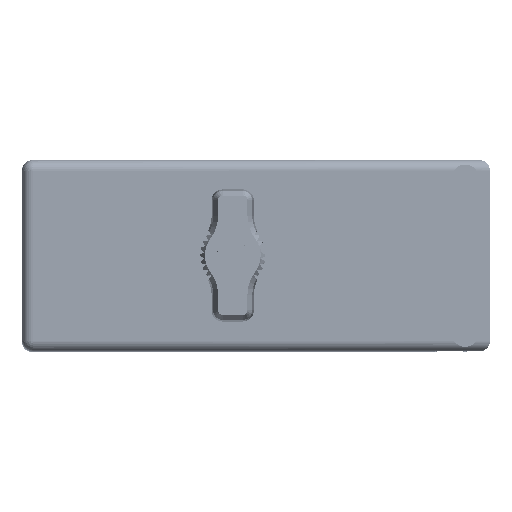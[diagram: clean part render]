
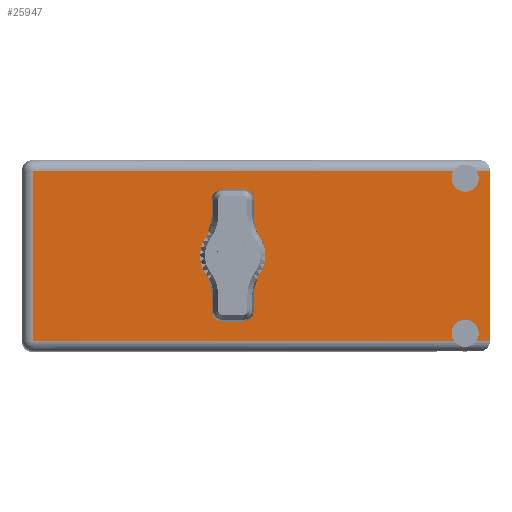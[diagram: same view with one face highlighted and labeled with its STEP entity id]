
A CAD part, top view. The second image highlights one B-rep face of the part: STEP entity #25947.
In plain terms, the highlighted face is planar.
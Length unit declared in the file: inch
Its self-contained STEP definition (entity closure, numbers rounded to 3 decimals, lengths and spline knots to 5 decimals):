
#608 = EDGE_CURVE ( 'NONE', #64827, #43503, #43738, .T. ) ;
#1348 = ORIENTED_EDGE ( 'NONE', *, *, #72574, .F. ) ;
#2503 = CARTESIAN_POINT ( 'NONE',  ( 2.858, 1.775, -1.117 ) ) ;
#2552 = EDGE_CURVE ( 'NONE', #55815, #45281, #53048, .T. ) ;
#5391 = EDGE_CURVE ( 'NONE', #49593, #26605, #30068, .T. ) ;
#7016 = CARTESIAN_POINT ( 'NONE',  ( 1.359, 1.775, -0.742 ) ) ;
#7832 = VERTEX_POINT ( 'NONE', #7016 ) ;
#7969 = DIRECTION ( 'NONE',  ( 0., 1., 0. ) ) ;
#9832 = DIRECTION ( 'NONE',  ( 0., 0., 1. ) ) ;
#10284 = CARTESIAN_POINT ( 'NONE',  ( 3.018, 1.775, -0.07 ) ) ;
#10767 = DIRECTION ( 'NONE',  ( 0., 1., 0. ) ) ;
#10955 = CARTESIAN_POINT ( 'NONE',  ( 2.78419, 1.775, -0.07 ) ) ;
#11032 = CARTESIAN_POINT ( 'NONE',  ( 0., 1.775, -1.164 ) ) ;
#12153 = VERTEX_POINT ( 'NONE', #41009 ) ;
#12749 = LINE ( 'NONE', #25932, #21412 ) ;
#14226 = VERTEX_POINT ( 'NONE', #76802 ) ;
#15541 = CARTESIAN_POINT ( 'NONE',  ( 0., 1.775, -1.234 ) ) ;
#15867 = EDGE_LOOP ( 'NONE', ( #76653, #56327, #40020, #50385, #50510, #75709, #87005, #17679, #46593, #50415 ) ) ;
#16666 = CARTESIAN_POINT ( 'NONE',  ( 2.858, 1.775, -1.117 ) ) ;
#17679 = ORIENTED_EDGE ( 'NONE', *, *, #23216, .F. ) ;
#18230 = DIRECTION ( 'NONE',  ( 0., 0., 1. ) ) ;
#19751 = CARTESIAN_POINT ( 'NONE',  ( 2.858, 1.775, -0.2045 ) ) ;
#20551 = LINE ( 'NONE', #66817, #37761 ) ;
#21412 = VECTOR ( 'NONE', #59395, 39.37008 ) ;
#21891 = AXIS2_PLACEMENT_3D ( 'NONE', #16666, #84684, #18230 ) ;
#21928 = DIRECTION ( 'NONE',  ( 0., 0., 1. ) ) ;
#22637 = AXIS2_PLACEMENT_3D ( 'NONE', #57628, #30516, #30221 ) ;
#22793 = VERTEX_POINT ( 'NONE', #72732 ) ;
#23216 = EDGE_CURVE ( 'NONE', #35299, #14226, #62063, .T. ) ;
#23480 = CARTESIAN_POINT ( 'NONE',  ( 0.07, 1.775, -0.07 ) ) ;
#23585 = CARTESIAN_POINT ( 'NONE',  ( 1.359, 1.775, -0.617 ) ) ;
#23761 = CARTESIAN_POINT ( 'NONE',  ( 3.018, 1.775, -0.07 ) ) ;
#23885 = DIRECTION ( 'NONE',  ( 0., 1., 0. ) ) ;
#24625 = DIRECTION ( 'NONE',  ( -1., 0., 0. ) ) ;
#24783 = EDGE_CURVE ( 'NONE', #35299, #22793, #45577, .T. ) ;
#25428 = CARTESIAN_POINT ( 'NONE',  ( 3.018, 1.775, -0.07 ) ) ;
#25932 = CARTESIAN_POINT ( 'NONE',  ( 0.07, 1.775, -1.234 ) ) ;
#25947 = ADVANCED_FACE ( 'NONE', ( #63700, #45318 ), #55640, .T. ) ;
#26605 = VERTEX_POINT ( 'NONE', #72598 ) ;
#26608 = CARTESIAN_POINT ( 'NONE',  ( 0., 1.775, -1.164 ) ) ;
#27994 = EDGE_CURVE ( 'NONE', #7832, #12153, #41611, .T. ) ;
#30068 = LINE ( 'NONE', #26608, #33294 ) ;
#30221 = DIRECTION ( 'NONE',  ( 0., 0., 1. ) ) ;
#30516 = DIRECTION ( 'NONE',  ( 0., 1., 0. ) ) ;
#31467 = AXIS2_PLACEMENT_3D ( 'NONE', #60810, #88711, #53539 ) ;
#32338 = DIRECTION ( 'NONE',  ( 1., 0., 0. ) ) ;
#32915 = CIRCLE ( 'NONE', #31467, 0.125 ) ;
#33294 = VECTOR ( 'NONE', #47387, 39.37008 ) ;
#33618 = CIRCLE ( 'NONE', #22637, 0.0875 ) ;
#35299 = VERTEX_POINT ( 'NONE', #47655 ) ;
#35574 = EDGE_LOOP ( 'NONE', ( #1348, #53172 ) ) ;
#36454 = CARTESIAN_POINT ( 'NONE',  ( 2.93181, 1.775, -0.07 ) ) ;
#37761 = VECTOR ( 'NONE', #59863, 39.37008 ) ;
#37840 = VERTEX_POINT ( 'NONE', #19751 ) ;
#40020 = ORIENTED_EDGE ( 'NONE', *, *, #79323, .F. ) ;
#41009 = CARTESIAN_POINT ( 'NONE',  ( 1.359, 1.775, -0.492 ) ) ;
#41571 = EDGE_CURVE ( 'NONE', #14226, #26605, #48069, .T. ) ;
#41611 = CIRCLE ( 'NONE', #65567, 0.125 ) ;
#42751 = EDGE_CURVE ( 'NONE', #37840, #43503, #49966, .T. ) ;
#43496 = DIRECTION ( 'NONE',  ( 0., 0., 1. ) ) ;
#43503 = VERTEX_POINT ( 'NONE', #10955 ) ;
#43738 = LINE ( 'NONE', #10284, #52410 ) ;
#45281 = VERTEX_POINT ( 'NONE', #23761 ) ;
#45318 = FACE_OUTER_BOUND ( 'NONE', #15867, .T. ) ;
#45577 = LINE ( 'NONE', #11032, #68267 ) ;
#46593 = ORIENTED_EDGE ( 'NONE', *, *, #24783, .T. ) ;
#47387 = DIRECTION ( 'NONE',  ( -1., 0., 0. ) ) ;
#47655 = CARTESIAN_POINT ( 'NONE',  ( 2.78419, 1.775, -1.164 ) ) ;
#48069 = CIRCLE ( 'NONE', #21891, 0.0875 ) ;
#49593 = VERTEX_POINT ( 'NONE', #88705 ) ;
#49966 = CIRCLE ( 'NONE', #69245, 0.0875 ) ;
#50385 = ORIENTED_EDGE ( 'NONE', *, *, #2552, .T. ) ;
#50415 = ORIENTED_EDGE ( 'NONE', *, *, #54622, .T. ) ;
#50510 = ORIENTED_EDGE ( 'NONE', *, *, #69260, .F. ) ;
#51152 = CARTESIAN_POINT ( 'NONE',  ( 2.858, 1.775, -0.117 ) ) ;
#52410 = VECTOR ( 'NONE', #32338, 39.37008 ) ;
#53048 = LINE ( 'NONE', #25428, #55197 ) ;
#53172 = ORIENTED_EDGE ( 'NONE', *, *, #27994, .F. ) ;
#53539 = DIRECTION ( 'NONE',  ( 0., 0., 1. ) ) ;
#54622 = EDGE_CURVE ( 'NONE', #22793, #64827, #12749, .T. ) ;
#55197 = VECTOR ( 'NONE', #81029, 39.37008 ) ;
#55640 = PLANE ( 'NONE',  #71692 ) ;
#55815 = VERTEX_POINT ( 'NONE', #36454 ) ;
#56327 = ORIENTED_EDGE ( 'NONE', *, *, #42751, .F. ) ;
#57082 = DIRECTION ( 'NONE',  ( 0., 1., 0. ) ) ;
#57628 = CARTESIAN_POINT ( 'NONE',  ( 2.858, 1.775, -0.117 ) ) ;
#59395 = DIRECTION ( 'NONE',  ( 0., 0., 1. ) ) ;
#59863 = DIRECTION ( 'NONE',  ( 0., 0., 1. ) ) ;
#60810 = CARTESIAN_POINT ( 'NONE',  ( 1.359, 1.775, -0.617 ) ) ;
#62063 = CIRCLE ( 'NONE', #79567, 0.0875 ) ;
#63700 = FACE_BOUND ( 'NONE', #35574, .T. ) ;
#64827 = VERTEX_POINT ( 'NONE', #23480 ) ;
#65567 = AXIS2_PLACEMENT_3D ( 'NONE', #23585, #23885, #85229 ) ;
#66817 = CARTESIAN_POINT ( 'NONE',  ( 3.018, 1.775, 0. ) ) ;
#68267 = VECTOR ( 'NONE', #24625, 39.37008 ) ;
#69245 = AXIS2_PLACEMENT_3D ( 'NONE', #51152, #10767, #9832 ) ;
#69260 = EDGE_CURVE ( 'NONE', #49593, #45281, #20551, .T. ) ;
#71692 = AXIS2_PLACEMENT_3D ( 'NONE', #15541, #7969, #21928 ) ;
#72574 = EDGE_CURVE ( 'NONE', #12153, #7832, #32915, .T. ) ;
#72598 = CARTESIAN_POINT ( 'NONE',  ( 2.93181, 1.775, -1.164 ) ) ;
#72732 = CARTESIAN_POINT ( 'NONE',  ( 0.07, 1.775, -1.164 ) ) ;
#75709 = ORIENTED_EDGE ( 'NONE', *, *, #5391, .T. ) ;
#76653 = ORIENTED_EDGE ( 'NONE', *, *, #608, .T. ) ;
#76802 = CARTESIAN_POINT ( 'NONE',  ( 2.858, 1.775, -1.0295 ) ) ;
#79323 = EDGE_CURVE ( 'NONE', #55815, #37840, #33618, .T. ) ;
#79567 = AXIS2_PLACEMENT_3D ( 'NONE', #2503, #57082, #43496 ) ;
#81029 = DIRECTION ( 'NONE',  ( 1., 0., 0. ) ) ;
#84684 = DIRECTION ( 'NONE',  ( 0., 1., 0. ) ) ;
#85229 = DIRECTION ( 'NONE',  ( 0., 0., 1. ) ) ;
#87005 = ORIENTED_EDGE ( 'NONE', *, *, #41571, .F. ) ;
#88705 = CARTESIAN_POINT ( 'NONE',  ( 3.018, 1.775, -1.164 ) ) ;
#88711 = DIRECTION ( 'NONE',  ( 0., 1., 0. ) ) ;
